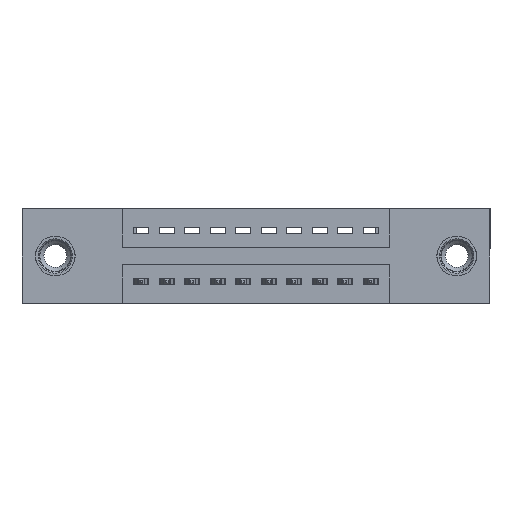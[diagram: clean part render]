
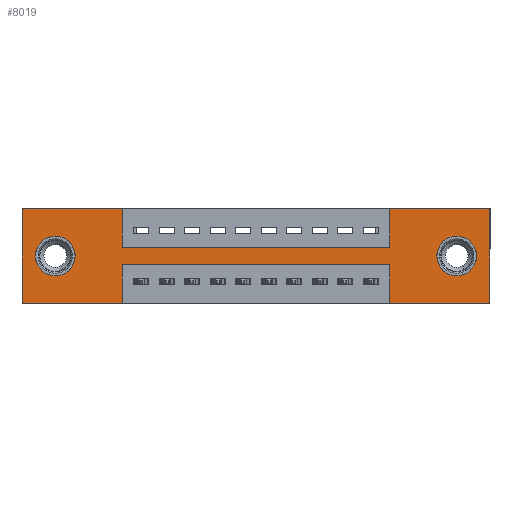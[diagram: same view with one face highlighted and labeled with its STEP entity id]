
A CAD part, front view. The second image highlights one B-rep face of the part: STEP entity #8019.
In plain terms, the highlighted planar face has unit normal (0, -1, 0).
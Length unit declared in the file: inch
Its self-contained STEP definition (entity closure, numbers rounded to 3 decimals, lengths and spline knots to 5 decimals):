
#52 = LINE ( 'NONE', #429, #9834 ) ;
#201 = DIRECTION ( 'NONE',  ( 1., 0., 0. ) ) ;
#229 = CARTESIAN_POINT ( 'NONE',  ( 0.3925, 0., -0.22 ) ) ;
#325 = DIRECTION ( 'NONE',  ( 0., 1., 0. ) ) ;
#429 = CARTESIAN_POINT ( 'NONE',  ( 0., 0., 0. ) ) ;
#630 = ORIENTED_EDGE ( 'NONE', *, *, #4132, .T. ) ;
#771 = CARTESIAN_POINT ( 'NONE',  ( 1.835, 0., 0. ) ) ;
#832 = EDGE_CURVE ( 'NONE', #7165, #11719, #10033, .T. ) ;
#836 = CARTESIAN_POINT ( 'NONE',  ( 1.4425, 0., 0. ) ) ;
#946 = LINE ( 'NONE', #2888, #3306 ) ;
#965 = DIRECTION ( 'NONE',  ( -1., 0., 0. ) ) ;
#966 = EDGE_CURVE ( 'NONE', #12530, #10517, #5142, .T. ) ;
#1433 = CARTESIAN_POINT ( 'NONE',  ( 0.13, 0., -0.107 ) ) ;
#1452 = VECTOR ( 'NONE', #5392, 39.37008 ) ;
#1519 = ORIENTED_EDGE ( 'NONE', *, *, #5512, .T. ) ;
#1772 = LINE ( 'NONE', #8243, #13948 ) ;
#2012 = DIRECTION ( 'NONE',  ( 0., 0., 1. ) ) ;
#2101 = VERTEX_POINT ( 'NONE', #5375 ) ;
#2408 = DIRECTION ( 'NONE',  ( 1., 0., 0. ) ) ;
#2415 = AXIS2_PLACEMENT_3D ( 'NONE', #6557, #3303, #10670 ) ;
#2558 = CARTESIAN_POINT ( 'NONE',  ( 1.4425, 0., -0.37 ) ) ;
#2594 = AXIS2_PLACEMENT_3D ( 'NONE', #3111, #12709, #9417 ) ;
#2643 = CIRCLE ( 'NONE', #2415, 0.078 ) ;
#2654 = DIRECTION ( 'NONE',  ( 0., 0., -1. ) ) ;
#2659 = ORIENTED_EDGE ( 'NONE', *, *, #832, .F. ) ;
#2776 = EDGE_LOOP ( 'NONE', ( #630, #1519 ) ) ;
#2846 = VERTEX_POINT ( 'NONE', #9827 ) ;
#2888 = CARTESIAN_POINT ( 'NONE',  ( 1.835, 0., 0. ) ) ;
#2994 = VERTEX_POINT ( 'NONE', #771 ) ;
#3019 = CARTESIAN_POINT ( 'NONE',  ( 0., 0., 0. ) ) ;
#3082 = DIRECTION ( 'NONE',  ( 1., 0., 0. ) ) ;
#3111 = CARTESIAN_POINT ( 'NONE',  ( 1.705, 0., -0.185 ) ) ;
#3175 = ORIENTED_EDGE ( 'NONE', *, *, #8677, .T. ) ;
#3303 = DIRECTION ( 'NONE',  ( 0., 1., 0. ) ) ;
#3306 = VECTOR ( 'NONE', #2654, 39.37008 ) ;
#3356 = AXIS2_PLACEMENT_3D ( 'NONE', #4856, #8103, #12536 ) ;
#3380 = ORIENTED_EDGE ( 'NONE', *, *, #7759, .F. ) ;
#3403 = CARTESIAN_POINT ( 'NONE',  ( 1.4425, 0., -0.22 ) ) ;
#3424 = AXIS2_PLACEMENT_3D ( 'NONE', #6793, #325, #8890 ) ;
#3500 = LINE ( 'NONE', #5718, #9371 ) ;
#3597 = VERTEX_POINT ( 'NONE', #2558 ) ;
#4008 = VECTOR ( 'NONE', #8651, 39.37008 ) ;
#4021 = VECTOR ( 'NONE', #2012, 39.37008 ) ;
#4132 = EDGE_CURVE ( 'NONE', #10293, #11391, #7061, .T. ) ;
#4411 = ORIENTED_EDGE ( 'NONE', *, *, #966, .F. ) ;
#4588 = EDGE_CURVE ( 'NONE', #2846, #3597, #12653, .T. ) ;
#4679 = EDGE_CURVE ( 'NONE', #12981, #13768, #13834, .T. ) ;
#4750 = DIRECTION ( 'NONE',  ( 0., 0., 1. ) ) ;
#4856 = CARTESIAN_POINT ( 'NONE',  ( 1.705, 0., -0.185 ) ) ;
#5122 = VECTOR ( 'NONE', #4750, 39.37008 ) ;
#5142 = LINE ( 'NONE', #6388, #1452 ) ;
#5216 = EDGE_CURVE ( 'NONE', #2101, #9808, #7020, .T. ) ;
#5253 = DIRECTION ( 'NONE',  ( 0., -1., 0. ) ) ;
#5375 = CARTESIAN_POINT ( 'NONE',  ( 1.705, 0., -0.263 ) ) ;
#5392 = DIRECTION ( 'NONE',  ( 0., 0., 1. ) ) ;
#5440 = CARTESIAN_POINT ( 'NONE',  ( 0.3925, 0., -0.37 ) ) ;
#5468 = DIRECTION ( 'NONE',  ( 0., 0., -1. ) ) ;
#5512 = EDGE_CURVE ( 'NONE', #11391, #10293, #2643, .T. ) ;
#5573 = EDGE_LOOP ( 'NONE', ( #3175, #5678 ) ) ;
#5639 = LINE ( 'NONE', #13506, #5122 ) ;
#5678 = ORIENTED_EDGE ( 'NONE', *, *, #5216, .T. ) ;
#5704 = EDGE_CURVE ( 'NONE', #13192, #7332, #5866, .T. ) ;
#5718 = CARTESIAN_POINT ( 'NONE',  ( 0.3925, 0., -0.15 ) ) ;
#5757 = ORIENTED_EDGE ( 'NONE', *, *, #9274, .F. ) ;
#5760 = EDGE_CURVE ( 'NONE', #7332, #12530, #7535, .T. ) ;
#5866 = LINE ( 'NONE', #8396, #11274 ) ;
#5931 = VECTOR ( 'NONE', #7350, 39.37008 ) ;
#6007 = CARTESIAN_POINT ( 'NONE',  ( 0.3925, 0., 0. ) ) ;
#6249 = CARTESIAN_POINT ( 'NONE',  ( 0., 0., -0.37 ) ) ;
#6250 = LINE ( 'NONE', #11748, #5931 ) ;
#6388 = CARTESIAN_POINT ( 'NONE',  ( 0., 0., 0. ) ) ;
#6435 = CARTESIAN_POINT ( 'NONE',  ( 0.13, 0., -0.263 ) ) ;
#6557 = CARTESIAN_POINT ( 'NONE',  ( 0.13, 0., -0.185 ) ) ;
#6632 = FACE_BOUND ( 'NONE', #5573, .T. ) ;
#6793 = CARTESIAN_POINT ( 'NONE',  ( 0.13, 0., -0.185 ) ) ;
#7020 = CIRCLE ( 'NONE', #2594, 0.078 ) ;
#7061 = CIRCLE ( 'NONE', #3424, 0.078 ) ;
#7090 = EDGE_CURVE ( 'NONE', #10517, #7165, #1772, .T. ) ;
#7165 = VERTEX_POINT ( 'NONE', #6007 ) ;
#7332 = VERTEX_POINT ( 'NONE', #5440 ) ;
#7350 = DIRECTION ( 'NONE',  ( -1., 0., 0. ) ) ;
#7477 = DIRECTION ( 'NONE',  ( 0., 0., -1. ) ) ;
#7535 = LINE ( 'NONE', #10868, #4008 ) ;
#7576 = ORIENTED_EDGE ( 'NONE', *, *, #7090, .F. ) ;
#7759 = EDGE_CURVE ( 'NONE', #3597, #13217, #5639, .T. ) ;
#7851 = EDGE_CURVE ( 'NONE', #13768, #2994, #52, .T. ) ;
#8019 = ADVANCED_FACE ( 'NONE', ( #6632, #9136, #10002 ), #12928, .T. ) ;
#8103 = DIRECTION ( 'NONE',  ( 0., 1., 0. ) ) ;
#8243 = CARTESIAN_POINT ( 'NONE',  ( 0., 0., 0. ) ) ;
#8396 = CARTESIAN_POINT ( 'NONE',  ( 0.3925, 0., -0.37 ) ) ;
#8651 = DIRECTION ( 'NONE',  ( -1., 0., 0. ) ) ;
#8677 = EDGE_CURVE ( 'NONE', #9808, #2101, #9294, .T. ) ;
#8746 = ORIENTED_EDGE ( 'NONE', *, *, #4679, .F. ) ;
#8800 = ORIENTED_EDGE ( 'NONE', *, *, #10179, .F. ) ;
#8869 = CARTESIAN_POINT ( 'NONE',  ( 1.705, 0., -0.107 ) ) ;
#8890 = DIRECTION ( 'NONE',  ( 0., 0., 1. ) ) ;
#9127 = ORIENTED_EDGE ( 'NONE', *, *, #7851, .F. ) ;
#9136 = FACE_BOUND ( 'NONE', #2776, .T. ) ;
#9274 = EDGE_CURVE ( 'NONE', #13217, #13192, #6250, .T. ) ;
#9294 = CIRCLE ( 'NONE', #3356, 0.078 ) ;
#9371 = VECTOR ( 'NONE', #2408, 39.37008 ) ;
#9417 = DIRECTION ( 'NONE',  ( 0., 0., -1. ) ) ;
#9662 = CARTESIAN_POINT ( 'NONE',  ( 0., 0., -0.37 ) ) ;
#9808 = VERTEX_POINT ( 'NONE', #8869 ) ;
#9827 = CARTESIAN_POINT ( 'NONE',  ( 1.835, 0., -0.37 ) ) ;
#9834 = VECTOR ( 'NONE', #201, 39.37008 ) ;
#10002 = FACE_OUTER_BOUND ( 'NONE', #10635, .T. ) ;
#10033 = LINE ( 'NONE', #12076, #11409 ) ;
#10152 = CARTESIAN_POINT ( 'NONE',  ( 0.3925, 0., -0.15 ) ) ;
#10179 = EDGE_CURVE ( 'NONE', #2994, #2846, #946, .T. ) ;
#10293 = VERTEX_POINT ( 'NONE', #1433 ) ;
#10517 = VERTEX_POINT ( 'NONE', #3019 ) ;
#10635 = EDGE_LOOP ( 'NONE', ( #12564, #5757, #3380, #13636, #8800, #9127, #8746, #10982, #2659, #7576, #4411, #12433 ) ) ;
#10670 = DIRECTION ( 'NONE',  ( 0., 0., 1. ) ) ;
#10822 = CARTESIAN_POINT ( 'NONE',  ( 0., 0., -0.37 ) ) ;
#10868 = CARTESIAN_POINT ( 'NONE',  ( 0., 0., -0.37 ) ) ;
#10982 = ORIENTED_EDGE ( 'NONE', *, *, #12252, .F. ) ;
#11274 = VECTOR ( 'NONE', #7477, 39.37008 ) ;
#11391 = VERTEX_POINT ( 'NONE', #6435 ) ;
#11409 = VECTOR ( 'NONE', #5468, 39.37008 ) ;
#11487 = AXIS2_PLACEMENT_3D ( 'NONE', #10822, #5253, #12825 ) ;
#11496 = CARTESIAN_POINT ( 'NONE',  ( 1.4425, 0., -0.15 ) ) ;
#11719 = VERTEX_POINT ( 'NONE', #10152 ) ;
#11748 = CARTESIAN_POINT ( 'NONE',  ( 0.3925, 0., -0.22 ) ) ;
#12076 = CARTESIAN_POINT ( 'NONE',  ( 0.3925, 0., 0. ) ) ;
#12252 = EDGE_CURVE ( 'NONE', #11719, #12981, #3500, .T. ) ;
#12433 = ORIENTED_EDGE ( 'NONE', *, *, #5760, .F. ) ;
#12530 = VERTEX_POINT ( 'NONE', #9662 ) ;
#12536 = DIRECTION ( 'NONE',  ( 0., 0., -1. ) ) ;
#12564 = ORIENTED_EDGE ( 'NONE', *, *, #5704, .F. ) ;
#12653 = LINE ( 'NONE', #6249, #12994 ) ;
#12709 = DIRECTION ( 'NONE',  ( 0., 1., 0. ) ) ;
#12825 = DIRECTION ( 'NONE',  ( 0., 0., -1. ) ) ;
#12928 = PLANE ( 'NONE',  #11487 ) ;
#12981 = VERTEX_POINT ( 'NONE', #11496 ) ;
#12994 = VECTOR ( 'NONE', #965, 39.37008 ) ;
#13192 = VERTEX_POINT ( 'NONE', #229 ) ;
#13217 = VERTEX_POINT ( 'NONE', #3403 ) ;
#13291 = CARTESIAN_POINT ( 'NONE',  ( 1.4425, 0., 0. ) ) ;
#13506 = CARTESIAN_POINT ( 'NONE',  ( 1.4425, 0., -0.37 ) ) ;
#13636 = ORIENTED_EDGE ( 'NONE', *, *, #4588, .F. ) ;
#13768 = VERTEX_POINT ( 'NONE', #13291 ) ;
#13834 = LINE ( 'NONE', #836, #4021 ) ;
#13948 = VECTOR ( 'NONE', #3082, 39.37008 ) ;
